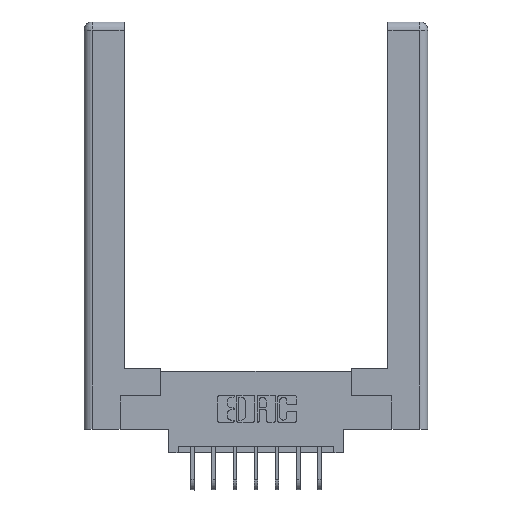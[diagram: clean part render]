
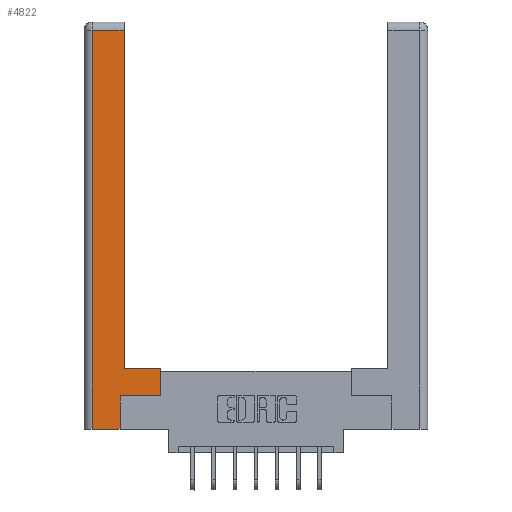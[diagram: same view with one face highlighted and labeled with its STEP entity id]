
A CAD part, top view. The second image highlights one B-rep face of the part: STEP entity #4822.
In plain terms, the highlighted planar face has unit normal (0, 0, 1).
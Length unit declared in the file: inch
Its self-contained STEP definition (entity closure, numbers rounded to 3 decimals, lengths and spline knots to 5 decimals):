
#373 = VERTEX_POINT ( 'NONE', #8938 ) ;
#391 = VERTEX_POINT ( 'NONE', #3656 ) ;
#968 = VECTOR ( 'NONE', #1700, 39.37008 ) ;
#1204 = ORIENTED_EDGE ( 'NONE', *, *, #8742, .T. ) ;
#1463 = CARTESIAN_POINT ( 'NONE',  ( 0.265, 0., 0. ) ) ;
#1700 = DIRECTION ( 'NONE',  ( 0., 1., 0. ) ) ;
#2198 = CARTESIAN_POINT ( 'NONE',  ( 0.265, 0., 0. ) ) ;
#2235 = EDGE_LOOP ( 'NONE', ( #8400, #1204, #5581, #5544, #8858, #5965, #6618, #8783 ) ) ;
#2352 = EDGE_CURVE ( 'NONE', #11255, #391, #5519, .T. ) ;
#2354 = VERTEX_POINT ( 'NONE', #7873 ) ;
#2417 = VERTEX_POINT ( 'NONE', #2198 ) ;
#2462 = LINE ( 'NONE', #5896, #11752 ) ;
#2603 = CARTESIAN_POINT ( 'NONE',  ( 0.565, 0.245, 0. ) ) ;
#2661 = CARTESIAN_POINT ( 'NONE',  ( 0., 0., 0. ) ) ;
#2702 = VERTEX_POINT ( 'NONE', #7606 ) ;
#3656 = CARTESIAN_POINT ( 'NONE',  ( 0.565, 0.45, 0. ) ) ;
#4159 = EDGE_CURVE ( 'NONE', #2702, #4634, #6436, .T. ) ;
#4170 = VECTOR ( 'NONE', #7609, 39.37008 ) ;
#4189 = VERTEX_POINT ( 'NONE', #4649 ) ;
#4234 = EDGE_CURVE ( 'NONE', #2354, #4189, #10093, .T. ) ;
#4397 = VECTOR ( 'NONE', #9641, 39.37008 ) ;
#4464 = EDGE_CURVE ( 'NONE', #373, #11255, #2462, .T. ) ;
#4621 = AXIS2_PLACEMENT_3D ( 'NONE', #2661, #11361, #11497 ) ;
#4634 = VERTEX_POINT ( 'NONE', #10191 ) ;
#4642 = DIRECTION ( 'NONE',  ( -1., 0., 0. ) ) ;
#4649 = CARTESIAN_POINT ( 'NONE',  ( 0.295, 2.94, 0. ) ) ;
#4686 = CARTESIAN_POINT ( 'NONE',  ( 0.0615, 2.94, 0. ) ) ;
#4822 = ADVANCED_FACE ( 'NONE', ( #6887 ), #5598, .F. ) ;
#5519 = LINE ( 'NONE', #10756, #9785 ) ;
#5544 = ORIENTED_EDGE ( 'NONE', *, *, #10708, .T. ) ;
#5581 = ORIENTED_EDGE ( 'NONE', *, *, #4159, .T. ) ;
#5598 = PLANE ( 'NONE',  #4621 ) ;
#5896 = CARTESIAN_POINT ( 'NONE',  ( 0.565, 0.245, 0. ) ) ;
#5965 = ORIENTED_EDGE ( 'NONE', *, *, #4464, .T. ) ;
#6018 = DIRECTION ( 'NONE',  ( 1., 0., 0. ) ) ;
#6166 = LINE ( 'NONE', #4686, #11502 ) ;
#6436 = LINE ( 'NONE', #11512, #4170 ) ;
#6618 = ORIENTED_EDGE ( 'NONE', *, *, #2352, .T. ) ;
#6887 = FACE_OUTER_BOUND ( 'NONE', #2235, .T. ) ;
#6929 = DIRECTION ( 'NONE',  ( 0., 1., 0. ) ) ;
#7192 = LINE ( 'NONE', #9304, #9795 ) ;
#7437 = EDGE_CURVE ( 'NONE', #391, #2354, #12583, .T. ) ;
#7477 = LINE ( 'NONE', #1463, #9772 ) ;
#7606 = CARTESIAN_POINT ( 'NONE',  ( 0.0615, 2.94, 0. ) ) ;
#7609 = DIRECTION ( 'NONE',  ( 0., -1., 0. ) ) ;
#7873 = CARTESIAN_POINT ( 'NONE',  ( 0.295, 0.45, 0. ) ) ;
#8388 = DIRECTION ( 'NONE',  ( 1., 0., 0. ) ) ;
#8400 = ORIENTED_EDGE ( 'NONE', *, *, #4234, .T. ) ;
#8414 = CARTESIAN_POINT ( 'NONE',  ( 0.295, 3., 0. ) ) ;
#8742 = EDGE_CURVE ( 'NONE', #4189, #2702, #6166, .T. ) ;
#8783 = ORIENTED_EDGE ( 'NONE', *, *, #7437, .T. ) ;
#8858 = ORIENTED_EDGE ( 'NONE', *, *, #10057, .T. ) ;
#8938 = CARTESIAN_POINT ( 'NONE',  ( 0.265, 0.245, 0. ) ) ;
#9213 = DIRECTION ( 'NONE',  ( 0., 1., 0. ) ) ;
#9304 = CARTESIAN_POINT ( 'NONE',  ( 0.265, 0.245, 0. ) ) ;
#9641 = DIRECTION ( 'NONE',  ( -1., 0., 0. ) ) ;
#9772 = VECTOR ( 'NONE', #8388, 39.37008 ) ;
#9785 = VECTOR ( 'NONE', #6929, 39.37008 ) ;
#9795 = VECTOR ( 'NONE', #9213, 39.37008 ) ;
#10057 = EDGE_CURVE ( 'NONE', #2417, #373, #7192, .T. ) ;
#10093 = LINE ( 'NONE', #8414, #968 ) ;
#10191 = CARTESIAN_POINT ( 'NONE',  ( 0.0615, 0., 0. ) ) ;
#10708 = EDGE_CURVE ( 'NONE', #4634, #2417, #7477, .T. ) ;
#10756 = CARTESIAN_POINT ( 'NONE',  ( 0.565, 0.45, 0. ) ) ;
#11255 = VERTEX_POINT ( 'NONE', #2603 ) ;
#11361 = DIRECTION ( 'NONE',  ( 0., 0., -1. ) ) ;
#11497 = DIRECTION ( 'NONE',  ( -1., 0., 0. ) ) ;
#11502 = VECTOR ( 'NONE', #4642, 39.37008 ) ;
#11512 = CARTESIAN_POINT ( 'NONE',  ( 0.0615, 0., 0. ) ) ;
#11585 = CARTESIAN_POINT ( 'NONE',  ( 0.295, 0.45, 0. ) ) ;
#11752 = VECTOR ( 'NONE', #6018, 39.37008 ) ;
#12583 = LINE ( 'NONE', #11585, #4397 ) ;
